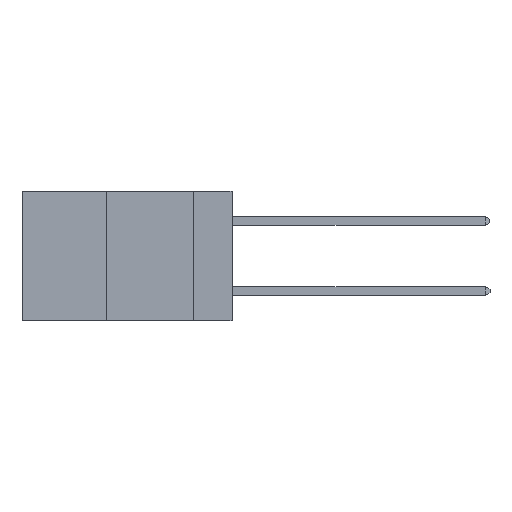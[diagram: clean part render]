
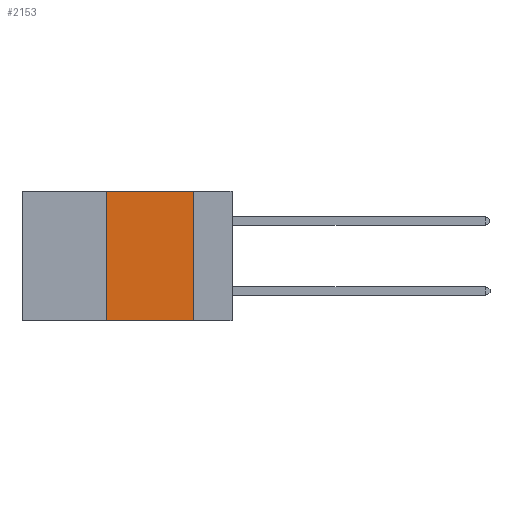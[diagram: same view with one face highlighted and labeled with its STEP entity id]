
A CAD part, left-side view. The second image highlights one B-rep face of the part: STEP entity #2153.
In plain terms, the highlighted planar face has unit normal (-1, 0, 0).
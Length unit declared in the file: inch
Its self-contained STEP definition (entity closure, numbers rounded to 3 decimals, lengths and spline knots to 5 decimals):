
#4 = PLANE ( 'NONE',  #11998 ) ;
#286 = VERTEX_POINT ( 'NONE', #10318 ) ;
#299 = VERTEX_POINT ( 'NONE', #10907 ) ;
#811 = EDGE_CURVE ( 'NONE', #299, #3384, #1628, .T. ) ;
#878 = ORIENTED_EDGE ( 'NONE', *, *, #3392, .F. ) ;
#1173 = DIRECTION ( 'NONE',  ( 1., 0., 0. ) ) ;
#1628 = LINE ( 'NONE', #4600, #9916 ) ;
#2000 = DIRECTION ( 'NONE',  ( 0., -1., 0. ) ) ;
#2153 = ADVANCED_FACE ( 'NONE', ( #13288 ), #4, .F. ) ;
#2268 = CARTESIAN_POINT ( 'NONE',  ( 0., 0.6, 0. ) ) ;
#2644 = VECTOR ( 'NONE', #2000, 39.37008 ) ;
#2780 = VECTOR ( 'NONE', #4378, 39.37008 ) ;
#3384 = VERTEX_POINT ( 'NONE', #10556 ) ;
#3392 = EDGE_CURVE ( 'NONE', #286, #299, #12139, .T. ) ;
#4378 = DIRECTION ( 'NONE',  ( 0., -1., 0. ) ) ;
#4461 = DIRECTION ( 'NONE',  ( 0., 0., -1. ) ) ;
#4499 = EDGE_CURVE ( 'NONE', #9146, #286, #8922, .T. ) ;
#4600 = CARTESIAN_POINT ( 'NONE',  ( 0., 0.11, 0. ) ) ;
#5488 = VECTOR ( 'NONE', #13256, 39.37008 ) ;
#5632 = EDGE_LOOP ( 'NONE', ( #9291, #878, #7189, #7517 ) ) ;
#5855 = EDGE_CURVE ( 'NONE', #9146, #3384, #11293, .T. ) ;
#6516 = CARTESIAN_POINT ( 'NONE',  ( 0., 0.6, -0.37 ) ) ;
#7189 = ORIENTED_EDGE ( 'NONE', *, *, #4499, .F. ) ;
#7517 = ORIENTED_EDGE ( 'NONE', *, *, #5855, .T. ) ;
#8858 = DIRECTION ( 'NONE',  ( 0., 0., -1. ) ) ;
#8922 = LINE ( 'NONE', #12216, #5488 ) ;
#9146 = VERTEX_POINT ( 'NONE', #9421 ) ;
#9291 = ORIENTED_EDGE ( 'NONE', *, *, #811, .F. ) ;
#9421 = CARTESIAN_POINT ( 'NONE',  ( 0., 0.36, -0.37 ) ) ;
#9916 = VECTOR ( 'NONE', #4461, 39.37008 ) ;
#10318 = CARTESIAN_POINT ( 'NONE',  ( 0., 0.36, 0. ) ) ;
#10556 = CARTESIAN_POINT ( 'NONE',  ( 0., 0.11, -0.37 ) ) ;
#10907 = CARTESIAN_POINT ( 'NONE',  ( 0., 0.11, 0. ) ) ;
#11293 = LINE ( 'NONE', #6516, #2780 ) ;
#11998 = AXIS2_PLACEMENT_3D ( 'NONE', #2268, #1173, #8858 ) ;
#12139 = LINE ( 'NONE', #12631, #2644 ) ;
#12216 = CARTESIAN_POINT ( 'NONE',  ( 0., 0.36, 0. ) ) ;
#12631 = CARTESIAN_POINT ( 'NONE',  ( 0., 0.6, 0. ) ) ;
#13256 = DIRECTION ( 'NONE',  ( 0., 0., 1. ) ) ;
#13288 = FACE_OUTER_BOUND ( 'NONE', #5632, .T. ) ;
